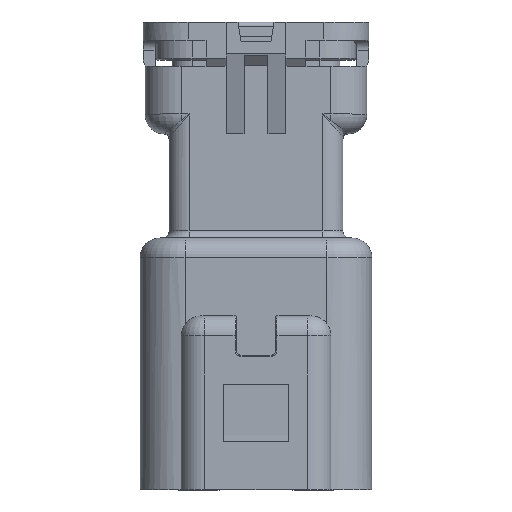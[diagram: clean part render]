
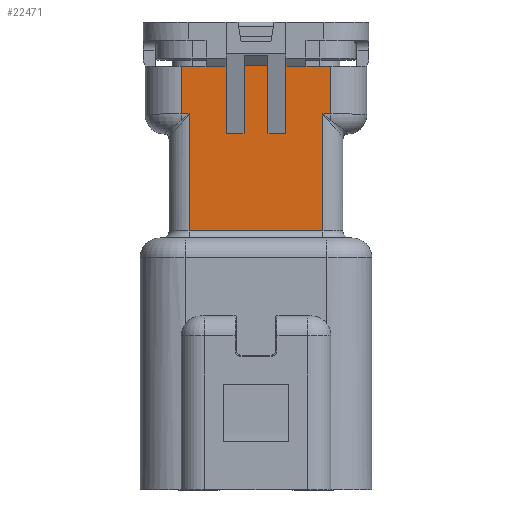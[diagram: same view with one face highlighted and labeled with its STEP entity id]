
A CAD part, top view. The second image highlights one B-rep face of the part: STEP entity #22471.
In plain terms, the highlighted planar face has unit normal (0, 0, 1).
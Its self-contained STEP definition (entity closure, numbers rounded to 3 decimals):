
#250 = VECTOR ( 'NONE', #10576, 1000. ) ;
#273 = VECTOR ( 'NONE', #20317, 1000. ) ;
#287 = VECTOR ( 'NONE', #12958, 1000. ) ;
#525 = ORIENTED_EDGE ( 'NONE', *, *, #21795, .F. ) ;
#612 = DIRECTION ( 'NONE',  ( 1., 0., 0. ) ) ;
#908 = EDGE_CURVE ( 'NONE', #23637, #11278, #8162, .T. ) ;
#1910 = VECTOR ( 'NONE', #8393, 1000. ) ;
#1952 = ORIENTED_EDGE ( 'NONE', *, *, #6279, .T. ) ;
#2707 = PLANE ( 'NONE',  #17821 ) ;
#2840 = CARTESIAN_POINT ( 'NONE',  ( 4.3, 23.4, 6.25 ) ) ;
#3111 = CARTESIAN_POINT ( 'NONE',  ( 0.25, 21.2, 6.25 ) ) ;
#3521 = CARTESIAN_POINT ( 'NONE',  ( 9.15, 18.8, 6.25 ) ) ;
#3602 = EDGE_CURVE ( 'NONE', #8480, #16378, #16577, .T. ) ;
#3710 = EDGE_CURVE ( 'NONE', #11386, #9374, #11947, .T. ) ;
#3802 = VERTEX_POINT ( 'NONE', #7920 ) ;
#3806 = LINE ( 'NONE', #13206, #16783 ) ;
#3872 = DIRECTION ( 'NONE',  ( 0., -1., 0. ) ) ;
#3971 = LINE ( 'NONE', #5795, #7672 ) ;
#4242 = VERTEX_POINT ( 'NONE', #10399 ) ;
#4338 = DIRECTION ( 'NONE',  ( 1., 0., 0. ) ) ;
#4665 = FACE_OUTER_BOUND ( 'NONE', #14375, .T. ) ;
#5099 = EDGE_CURVE ( 'NONE', #16378, #9256, #15961, .T. ) ;
#5380 = CARTESIAN_POINT ( 'NONE',  ( 6.4, 21.2, 6.25 ) ) ;
#5401 = CARTESIAN_POINT ( 'NONE',  ( 9.55, 18.8, 6.25 ) ) ;
#5434 = ORIENTED_EDGE ( 'NONE', *, *, #16352, .T. ) ;
#5795 = CARTESIAN_POINT ( 'NONE',  ( 9.55, 17.8, 6.25 ) ) ;
#6129 = CARTESIAN_POINT ( 'NONE',  ( 2.05, 21.2, 6.25 ) ) ;
#6147 = VECTOR ( 'NONE', #4338, 1000. ) ;
#6195 = LINE ( 'NONE', #10093, #7694 ) ;
#6279 = EDGE_CURVE ( 'NONE', #19957, #10869, #6195, .T. ) ;
#6425 = EDGE_CURVE ( 'NONE', #13718, #3802, #20075, .T. ) ;
#6456 = LINE ( 'NONE', #11588, #15539 ) ;
#6521 = LINE ( 'NONE', #21643, #9399 ) ;
#6724 = EDGE_CURVE ( 'NONE', #19590, #8601, #6521, .T. ) ;
#6747 = VECTOR ( 'NONE', #20417, 1000. ) ;
#7321 = CARTESIAN_POINT ( 'NONE',  ( 2.45, 18.8, 6.25 ) ) ;
#7670 = CARTESIAN_POINT ( 'NONE',  ( 4.3, 17.8, 6.25 ) ) ;
#7672 = VECTOR ( 'NONE', #9458, 1000. ) ;
#7694 = VECTOR ( 'NONE', #17410, 1000. ) ;
#7920 = CARTESIAN_POINT ( 'NONE',  ( 2.05, 18.8, 6.25 ) ) ;
#8162 = LINE ( 'NONE', #15838, #250 ) ;
#8393 = DIRECTION ( 'NONE',  ( 0., 1., 0. ) ) ;
#8429 = VERTEX_POINT ( 'NONE', #7321 ) ;
#8480 = VERTEX_POINT ( 'NONE', #23929 ) ;
#8601 = VERTEX_POINT ( 'NONE', #9532 ) ;
#9012 = EDGE_CURVE ( 'NONE', #19973, #23693, #15746, .T. ) ;
#9060 = CARTESIAN_POINT ( 'NONE',  ( 9.15, 12.95, 6.25 ) ) ;
#9164 = DIRECTION ( 'NONE',  ( 1., 0., 0. ) ) ;
#9256 = VERTEX_POINT ( 'NONE', #3521 ) ;
#9321 = ORIENTED_EDGE ( 'NONE', *, *, #5099, .T. ) ;
#9374 = VERTEX_POINT ( 'NONE', #21948 ) ;
#9399 = VECTOR ( 'NONE', #17979, 1000. ) ;
#9458 = DIRECTION ( 'NONE',  ( 0., 1., 0. ) ) ;
#9532 = CARTESIAN_POINT ( 'NONE',  ( 8.3, 21.2, 6.25 ) ) ;
#9943 = EDGE_CURVE ( 'NONE', #8429, #8480, #10306, .T. ) ;
#9989 = ORIENTED_EDGE ( 'NONE', *, *, #6425, .T. ) ;
#10093 = CARTESIAN_POINT ( 'NONE',  ( 1.45, 21.214, 6.25 ) ) ;
#10146 = DIRECTION ( 'NONE',  ( 0., 0., -1. ) ) ;
#10173 = VECTOR ( 'NONE', #17960, 1000. ) ;
#10306 = LINE ( 'NONE', #14219, #19855 ) ;
#10374 = CARTESIAN_POINT ( 'NONE',  ( 4.3, 21.2, 6.25 ) ) ;
#10399 = CARTESIAN_POINT ( 'NONE',  ( 7.3, 21.2, 6.25 ) ) ;
#10576 = DIRECTION ( 'NONE',  ( 1., 0., 0. ) ) ;
#10716 = CARTESIAN_POINT ( 'NONE',  ( 9.55, 21.2, 6.25 ) ) ;
#10806 = CARTESIAN_POINT ( 'NONE',  ( 6.4, 21.214, 6.25 ) ) ;
#10835 = DIRECTION ( 'NONE',  ( 1., 0., 0. ) ) ;
#10869 = VERTEX_POINT ( 'NONE', #16430 ) ;
#11278 = VERTEX_POINT ( 'NONE', #13001 ) ;
#11327 = VECTOR ( 'NONE', #21213, 1000. ) ;
#11386 = VERTEX_POINT ( 'NONE', #22989 ) ;
#11516 = ORIENTED_EDGE ( 'NONE', *, *, #9943, .T. ) ;
#11588 = CARTESIAN_POINT ( 'NONE',  ( 7.3, 23.4, 6.25 ) ) ;
#11888 = ORIENTED_EDGE ( 'NONE', *, *, #9012, .F. ) ;
#11947 = LINE ( 'NONE', #7670, #11327 ) ;
#12106 = CARTESIAN_POINT ( 'NONE',  ( 6.4, 17.8, 6.25 ) ) ;
#12228 = ORIENTED_EDGE ( 'NONE', *, *, #12708, .T. ) ;
#12708 = EDGE_CURVE ( 'NONE', #23637, #19957, #22344, .T. ) ;
#12958 = DIRECTION ( 'NONE',  ( 0., 1., 0. ) ) ;
#12987 = CARTESIAN_POINT ( 'NONE',  ( 1.45, 18.8, 6.25 ) ) ;
#13001 = CARTESIAN_POINT ( 'NONE',  ( 7.3, 17.8, 6.25 ) ) ;
#13206 = CARTESIAN_POINT ( 'NONE',  ( 1.45, 18.8, 6.25 ) ) ;
#13277 = ORIENTED_EDGE ( 'NONE', *, *, #14020, .F. ) ;
#13279 = EDGE_CURVE ( 'NONE', #13718, #19973, #15792, .T. ) ;
#13561 = VERTEX_POINT ( 'NONE', #5401 ) ;
#13718 = VERTEX_POINT ( 'NONE', #6129 ) ;
#13775 = ORIENTED_EDGE ( 'NONE', *, *, #21973, .T. ) ;
#13857 = CARTESIAN_POINT ( 'NONE',  ( 0.25, 21.2, 6.25 ) ) ;
#13889 = ORIENTED_EDGE ( 'NONE', *, *, #908, .F. ) ;
#13960 = LINE ( 'NONE', #2840, #10173 ) ;
#14020 = EDGE_CURVE ( 'NONE', #11278, #4242, #6456, .T. ) ;
#14219 = CARTESIAN_POINT ( 'NONE',  ( 2.45, 17.8, 6.25 ) ) ;
#14375 = EDGE_LOOP ( 'NONE', ( #9321, #19426, #13775, #22825, #525, #13277, #13889, #12228, #1952, #20224, #18998, #16527, #11888, #19150, #9989, #5434, #11516, #21302 ) ) ;
#14445 = LINE ( 'NONE', #12987, #6747 ) ;
#14735 = CARTESIAN_POINT ( 'NONE',  ( 3.3, 21.2, 6.25 ) ) ;
#15539 = VECTOR ( 'NONE', #15735, 1000. ) ;
#15735 = DIRECTION ( 'NONE',  ( 0., 1., 0. ) ) ;
#15746 = LINE ( 'NONE', #20754, #17629 ) ;
#15792 = LINE ( 'NONE', #13857, #6147 ) ;
#15838 = CARTESIAN_POINT ( 'NONE',  ( 4.3, 17.8, 6.25 ) ) ;
#15872 = CARTESIAN_POINT ( 'NONE',  ( 1.45, 17.8, 6.25 ) ) ;
#15961 = LINE ( 'NONE', #17668, #1910 ) ;
#16059 = DIRECTION ( 'NONE',  ( 0., -1., 0. ) ) ;
#16352 = EDGE_CURVE ( 'NONE', #3802, #8429, #14445, .T. ) ;
#16378 = VERTEX_POINT ( 'NONE', #9060 ) ;
#16430 = CARTESIAN_POINT ( 'NONE',  ( 5.2, 21.214, 6.25 ) ) ;
#16527 = ORIENTED_EDGE ( 'NONE', *, *, #19143, .F. ) ;
#16577 = LINE ( 'NONE', #20486, #21083 ) ;
#16646 = LINE ( 'NONE', #3111, #273 ) ;
#16783 = VECTOR ( 'NONE', #9164, 1000. ) ;
#17349 = DIRECTION ( 'NONE',  ( -1., 0., 0. ) ) ;
#17410 = DIRECTION ( 'NONE',  ( -1., 0., 0. ) ) ;
#17629 = VECTOR ( 'NONE', #612, 1000. ) ;
#17668 = CARTESIAN_POINT ( 'NONE',  ( 9.15, 17.8, 6.25 ) ) ;
#17817 = VECTOR ( 'NONE', #16059, 1000. ) ;
#17821 = AXIS2_PLACEMENT_3D ( 'NONE', #15872, #10146, #17349 ) ;
#17960 = DIRECTION ( 'NONE',  ( 0., -1., 0. ) ) ;
#17979 = DIRECTION ( 'NONE',  ( -1., 0., 0. ) ) ;
#18873 = CARTESIAN_POINT ( 'NONE',  ( 5.2, 21.2, 6.25 ) ) ;
#18998 = ORIENTED_EDGE ( 'NONE', *, *, #3710, .F. ) ;
#19143 = EDGE_CURVE ( 'NONE', #23693, #11386, #13960, .T. ) ;
#19150 = ORIENTED_EDGE ( 'NONE', *, *, #13279, .F. ) ;
#19231 = EDGE_CURVE ( 'NONE', #9256, #13561, #3806, .T. ) ;
#19426 = ORIENTED_EDGE ( 'NONE', *, *, #19231, .T. ) ;
#19590 = VERTEX_POINT ( 'NONE', #10716 ) ;
#19855 = VECTOR ( 'NONE', #21651, 1000. ) ;
#19957 = VERTEX_POINT ( 'NONE', #10806 ) ;
#19973 = VERTEX_POINT ( 'NONE', #14735 ) ;
#20075 = LINE ( 'NONE', #21554, #17817 ) ;
#20116 = VECTOR ( 'NONE', #3872, 1000. ) ;
#20224 = ORIENTED_EDGE ( 'NONE', *, *, #21573, .T. ) ;
#20317 = DIRECTION ( 'NONE',  ( 1., 0., 0. ) ) ;
#20417 = DIRECTION ( 'NONE',  ( 1., 0., 0. ) ) ;
#20486 = CARTESIAN_POINT ( 'NONE',  ( 1.45, 12.95, 6.25 ) ) ;
#20754 = CARTESIAN_POINT ( 'NONE',  ( 0.25, 21.2, 6.25 ) ) ;
#21083 = VECTOR ( 'NONE', #10835, 1000. ) ;
#21213 = DIRECTION ( 'NONE',  ( 1., 0., 0. ) ) ;
#21302 = ORIENTED_EDGE ( 'NONE', *, *, #3602, .T. ) ;
#21554 = CARTESIAN_POINT ( 'NONE',  ( 2.05, 17.8, 6.25 ) ) ;
#21573 = EDGE_CURVE ( 'NONE', #10869, #9374, #22782, .T. ) ;
#21643 = CARTESIAN_POINT ( 'NONE',  ( 1.45, 21.2, 6.25 ) ) ;
#21651 = DIRECTION ( 'NONE',  ( 0., -1., 0. ) ) ;
#21795 = EDGE_CURVE ( 'NONE', #4242, #8601, #16646, .T. ) ;
#21948 = CARTESIAN_POINT ( 'NONE',  ( 5.2, 17.8, 6.25 ) ) ;
#21973 = EDGE_CURVE ( 'NONE', #13561, #19590, #3971, .T. ) ;
#22344 = LINE ( 'NONE', #5380, #287 ) ;
#22471 = ADVANCED_FACE ( 'NONE', ( #4665 ), #2707, .F. ) ;
#22782 = LINE ( 'NONE', #18873, #20116 ) ;
#22825 = ORIENTED_EDGE ( 'NONE', *, *, #6724, .T. ) ;
#22989 = CARTESIAN_POINT ( 'NONE',  ( 4.3, 17.8, 6.25 ) ) ;
#23637 = VERTEX_POINT ( 'NONE', #12106 ) ;
#23693 = VERTEX_POINT ( 'NONE', #10374 ) ;
#23929 = CARTESIAN_POINT ( 'NONE',  ( 2.45, 12.95, 6.25 ) ) ;
